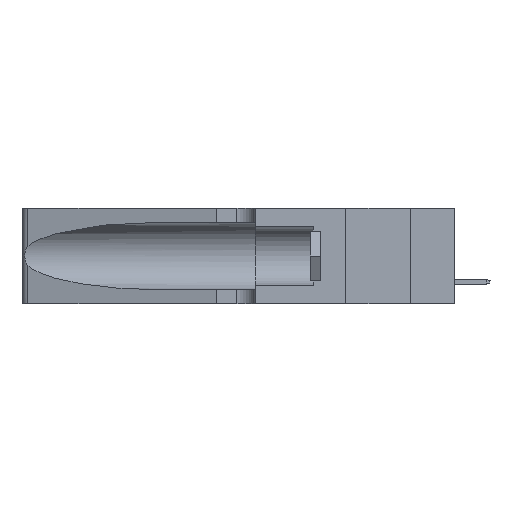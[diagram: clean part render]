
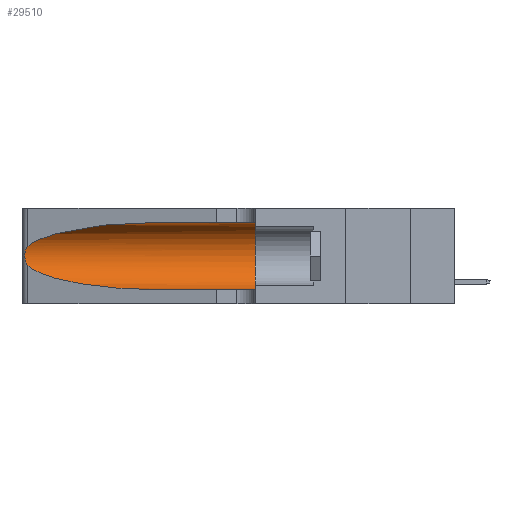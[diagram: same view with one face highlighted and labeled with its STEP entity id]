
A CAD part, left-side view. The second image highlights one B-rep face of the part: STEP entity #29510.
In plain terms, the highlighted cylindrical face has radius 3.308 mm (diameter 6.617 mm), a partial arc.
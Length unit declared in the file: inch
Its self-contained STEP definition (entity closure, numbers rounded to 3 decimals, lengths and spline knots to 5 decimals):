
#1299 = ORIENTED_EDGE ( 'NONE', *, *, #29385, .F. ) ;
#2077 = CARTESIAN_POINT ( 'NONE',  ( 0.18966, 0.96281, 0.31525 ) ) ;
#3329 = ORIENTED_EDGE ( 'NONE', *, *, #9801, .T. ) ;
#3937 = CARTESIAN_POINT ( 'NONE',  ( 0.1305, 0.72297, 0.31525 ) ) ;
#4186 = CARTESIAN_POINT ( 'NONE',  ( 0.25789, 1.23486, 0.15765 ) ) ;
#5390 = ORIENTED_EDGE ( 'NONE', *, *, #22626, .T. ) ;
#6193 = CARTESIAN_POINT ( 'NONE',  ( 0.1305, 0.72297, 0.05475 ) ) ;
#6408 = CARTESIAN_POINT ( 'NONE',  ( 0.2373, 1.15595, 0.08982 ) ) ;
#6502 = CARTESIAN_POINT ( 'NONE',  ( 0.25787, 1.23484, 0.2124 ) ) ;
#7282 = ORIENTED_EDGE ( 'NONE', *, *, #25850, .T. ) ;
#7655 = VERTEX_POINT ( 'NONE', #26781 ) ;
#7944 = CYLINDRICAL_SURFACE ( 'NONE', #15743, 0.13025 ) ;
#7985 = CARTESIAN_POINT ( 'NONE',  ( 0.1305, 0.35, 0.185 ) ) ;
#8004 = CARTESIAN_POINT ( 'NONE',  ( 0.1305, 1.61858, 0.05475 ) ) ;
#8649 = CARTESIAN_POINT ( 'NONE',  ( 0.26075, 1.23896, 0.178 ) ) ;
#8890 = LINE ( 'NONE', #30135, #17230 ) ;
#9098 = CARTESIAN_POINT ( 'NONE',  ( 0.25487, 1.22718, 0.22369 ) ) ;
#9238 = VECTOR ( 'NONE', #28799, 39.37008 ) ;
#9243 = CARTESIAN_POINT ( 'NONE',  ( 0.26017, 1.23833, 0.17102 ) ) ;
#9801 = EDGE_CURVE ( 'NONE', #18380, #7655, #13369, .T. ) ;
#10841 = VERTEX_POINT ( 'NONE', #6193 ) ;
#11563 = CARTESIAN_POINT ( 'NONE',  ( 0.25639, 1.23184, 0.21858 ) ) ;
#11574 =( BOUNDED_CURVE ( )  B_SPLINE_CURVE ( 3, ( #13761, #6408, #15746, #29976 ),
 .UNSPECIFIED., .F., .F. ) 
 B_SPLINE_CURVE_WITH_KNOTS ( ( 4, 4 ),
 ( 3.44316, 4.71239 ),
 .UNSPECIFIED. ) 
 CURVE ( )  GEOMETRIC_REPRESENTATION_ITEM ( )  RATIONAL_B_SPLINE_CURVE ( ( 1., 0.87, 0.87, 1. ) ) 
 REPRESENTATION_ITEM ( '' )  );
#13369 = B_SPLINE_CURVE_WITH_KNOTS ( 'NONE', 3,
 ( #9098, #18428, #11563, #6502, #27752, #20867, #23294, #8649, #9243, #25163, #4186, #15970, #13558, #25304 ),
 .UNSPECIFIED., .F., .F.,
 ( 4, 2, 2, 2, 2, 2, 4 ),
 ( 0., 0.00027, 0.00053, 0.00107, 0.0016, 0.00187, 0.00214 ),
 .UNSPECIFIED. ) ;
#13558 = CARTESIAN_POINT ( 'NONE',  ( 0.25555, 1.22993, 0.14849 ) ) ;
#13716 =( BOUNDED_CURVE ( )  B_SPLINE_CURVE ( 3, ( #3937, #2077, #27214, #18477 ),
 .UNSPECIFIED., .F., .F. ) 
 B_SPLINE_CURVE_WITH_KNOTS ( ( 4, 4 ),
 ( 1.5708, 2.84003 ),
 .UNSPECIFIED. ) 
 CURVE ( )  GEOMETRIC_REPRESENTATION_ITEM ( )  RATIONAL_B_SPLINE_CURVE ( ( 1., 0.87, 0.87, 1. ) ) 
 REPRESENTATION_ITEM ( '' )  );
#13761 = CARTESIAN_POINT ( 'NONE',  ( 0.25487, 1.22718, 0.14631 ) ) ;
#14535 = CARTESIAN_POINT ( 'NONE',  ( 0.1305, 0.35, 0.05475 ) ) ;
#15307 = CARTESIAN_POINT ( 'NONE',  ( 0.1305, 0.72297, 0.31525 ) ) ;
#15743 = AXIS2_PLACEMENT_3D ( 'NONE', #26310, #23983, #26457 ) ;
#15746 = CARTESIAN_POINT ( 'NONE',  ( 0.18966, 0.96281, 0.05475 ) ) ;
#15970 = CARTESIAN_POINT ( 'NONE',  ( 0.25639, 1.23186, 0.15144 ) ) ;
#16102 = EDGE_LOOP ( 'NONE', ( #5390, #3329, #27845, #7282, #29027, #1299 ) ) ;
#17179 = CIRCLE ( 'NONE', #23512, 0.13025 ) ;
#17230 = VECTOR ( 'NONE', #18378, 39.37008 ) ;
#17895 = VERTEX_POINT ( 'NONE', #14535 ) ;
#18116 = EDGE_CURVE ( 'NONE', #7655, #10841, #11574, .T. ) ;
#18378 = DIRECTION ( 'NONE',  ( 0., -1., 0. ) ) ;
#18380 = VERTEX_POINT ( 'NONE', #23958 ) ;
#18428 = CARTESIAN_POINT ( 'NONE',  ( 0.25555, 1.22994, 0.2215 ) ) ;
#18477 = CARTESIAN_POINT ( 'NONE',  ( 0.25487, 1.22718, 0.22369 ) ) ;
#20867 = CARTESIAN_POINT ( 'NONE',  ( 0.26018, 1.23835, 0.19895 ) ) ;
#21043 = VERTEX_POINT ( 'NONE', #25384 ) ;
#22626 = EDGE_CURVE ( 'NONE', #27944, #18380, #13716, .T. ) ;
#23294 = CARTESIAN_POINT ( 'NONE',  ( 0.26075, 1.23896, 0.19203 ) ) ;
#23512 = AXIS2_PLACEMENT_3D ( 'NONE', #7985, #26063, #24178 ) ;
#23958 = CARTESIAN_POINT ( 'NONE',  ( 0.25487, 1.22718, 0.22369 ) ) ;
#23983 = DIRECTION ( 'NONE',  ( 0., -1., 0. ) ) ;
#24178 = DIRECTION ( 'NONE',  ( 0., 0., 1. ) ) ;
#25163 = CARTESIAN_POINT ( 'NONE',  ( 0.25856, 1.23593, 0.16098 ) ) ;
#25304 = CARTESIAN_POINT ( 'NONE',  ( 0.25487, 1.22718, 0.14631 ) ) ;
#25384 = CARTESIAN_POINT ( 'NONE',  ( 0.1305, 0.35, 0.31525 ) ) ;
#25850 = EDGE_CURVE ( 'NONE', #10841, #17895, #29416, .T. ) ;
#26063 = DIRECTION ( 'NONE',  ( 0., 1., 0. ) ) ;
#26310 = CARTESIAN_POINT ( 'NONE',  ( 0.1305, 1.61858, 0.185 ) ) ;
#26457 = DIRECTION ( 'NONE',  ( 0., 0., -1. ) ) ;
#26781 = CARTESIAN_POINT ( 'NONE',  ( 0.25487, 1.22718, 0.14631 ) ) ;
#27214 = CARTESIAN_POINT ( 'NONE',  ( 0.2373, 1.15595, 0.28018 ) ) ;
#27752 = CARTESIAN_POINT ( 'NONE',  ( 0.25854, 1.2359, 0.20912 ) ) ;
#27845 = ORIENTED_EDGE ( 'NONE', *, *, #18116, .T. ) ;
#27944 = VERTEX_POINT ( 'NONE', #15307 ) ;
#28452 = FACE_OUTER_BOUND ( 'NONE', #16102, .T. ) ;
#28799 = DIRECTION ( 'NONE',  ( 0., -1., 0. ) ) ;
#29027 = ORIENTED_EDGE ( 'NONE', *, *, #29125, .F. ) ;
#29125 = EDGE_CURVE ( 'NONE', #21043, #17895, #17179, .T. ) ;
#29385 = EDGE_CURVE ( 'NONE', #27944, #21043, #8890, .T. ) ;
#29416 = LINE ( 'NONE', #8004, #9238 ) ;
#29510 = ADVANCED_FACE ( 'NONE', ( #28452 ), #7944, .F. ) ;
#29976 = CARTESIAN_POINT ( 'NONE',  ( 0.1305, 0.72297, 0.05475 ) ) ;
#30135 = CARTESIAN_POINT ( 'NONE',  ( 0.1305, 1.61858, 0.31525 ) ) ;
